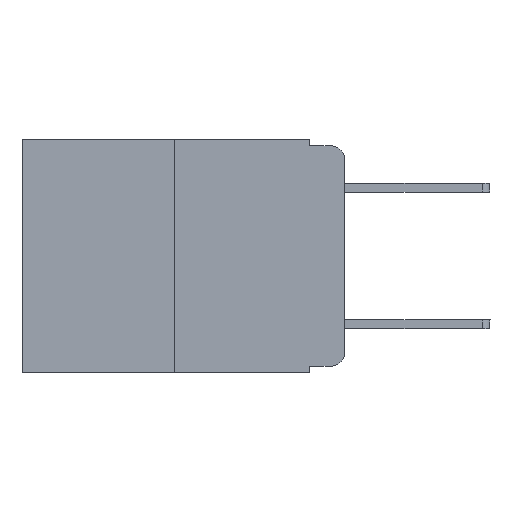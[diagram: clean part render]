
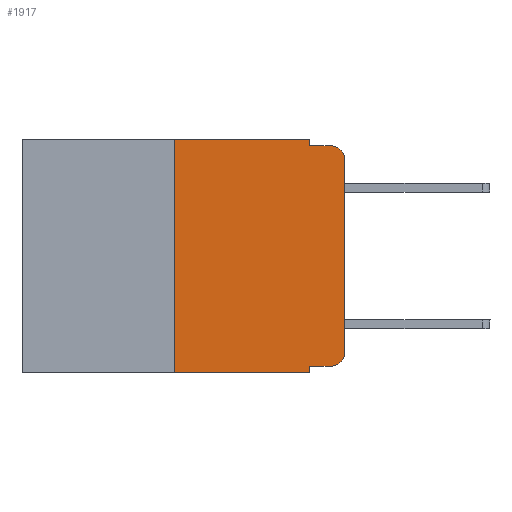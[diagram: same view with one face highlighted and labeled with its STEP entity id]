
A CAD part, left-side view. The second image highlights one B-rep face of the part: STEP entity #1917.
In plain terms, the highlighted planar face has unit normal (-1, 0, 0).
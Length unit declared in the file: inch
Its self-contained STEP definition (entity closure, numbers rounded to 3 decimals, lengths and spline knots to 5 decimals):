
#422 = CARTESIAN_POINT ( 'NONE',  ( 0., 0.02, -0.01 ) ) ;
#666 = ORIENTED_EDGE ( 'NONE', *, *, #4381, .T. ) ;
#1009 = CARTESIAN_POINT ( 'NONE',  ( 0., 0.051, 0. ) ) ;
#1027 = DIRECTION ( 'NONE',  ( 0., -1., 0. ) ) ;
#1063 = CARTESIAN_POINT ( 'NONE',  ( 0., 0.473, 0. ) ) ;
#1115 = ORIENTED_EDGE ( 'NONE', *, *, #6972, .F. ) ;
#1602 = PLANE ( 'NONE',  #3315 ) ;
#1678 = DIRECTION ( 'NONE',  ( 0., -1., 0. ) ) ;
#1718 = EDGE_CURVE ( 'NONE', #6401, #4799, #1751, .T. ) ;
#1751 = LINE ( 'NONE', #2748, #5522 ) ;
#1917 = ADVANCED_FACE ( 'NONE', ( #4671 ), #1602, .F. ) ;
#1966 = DIRECTION ( 'NONE',  ( 0., 0., -1. ) ) ;
#2652 = CARTESIAN_POINT ( 'NONE',  ( 0., 0.051, -0.01 ) ) ;
#2748 = CARTESIAN_POINT ( 'NONE',  ( 0., 0.473, -0.343 ) ) ;
#2893 = CIRCLE ( 'NONE', #5453, 0.02 ) ;
#3029 = VERTEX_POINT ( 'NONE', #7364 ) ;
#3074 = EDGE_CURVE ( 'NONE', #6401, #11103, #7754, .T. ) ;
#3315 = AXIS2_PLACEMENT_3D ( 'NONE', #6069, #7939, #7897 ) ;
#3561 = DIRECTION ( 'NONE',  ( 0., -1., 0. ) ) ;
#3565 = VERTEX_POINT ( 'NONE', #10255 ) ;
#3640 = VECTOR ( 'NONE', #1678, 39.37008 ) ;
#3647 = LINE ( 'NONE', #7190, #3640 ) ;
#3784 = CARTESIAN_POINT ( 'NONE',  ( 0., 0.25, 0. ) ) ;
#4093 = EDGE_CURVE ( 'NONE', #3565, #3029, #3647, .T. ) ;
#4182 = ORIENTED_EDGE ( 'NONE', *, *, #6627, .T. ) ;
#4257 = VERTEX_POINT ( 'NONE', #1009 ) ;
#4373 = DIRECTION ( 'NONE',  ( 0., 0., -1. ) ) ;
#4381 = EDGE_CURVE ( 'NONE', #5866, #6179, #5991, .T. ) ;
#4470 = LINE ( 'NONE', #5321, #10133 ) ;
#4671 = FACE_OUTER_BOUND ( 'NONE', #10088, .T. ) ;
#4758 = ORIENTED_EDGE ( 'NONE', *, *, #3074, .F. ) ;
#4799 = VERTEX_POINT ( 'NONE', #10731 ) ;
#4869 = LINE ( 'NONE', #2652, #9124 ) ;
#5321 = CARTESIAN_POINT ( 'NONE',  ( 0., 0.051, 0. ) ) ;
#5339 = CARTESIAN_POINT ( 'NONE',  ( 0., 0., -0.03 ) ) ;
#5453 = AXIS2_PLACEMENT_3D ( 'NONE', #11638, #9806, #4373 ) ;
#5522 = VECTOR ( 'NONE', #1027, 39.37008 ) ;
#5866 = VERTEX_POINT ( 'NONE', #5339 ) ;
#5936 = ORIENTED_EDGE ( 'NONE', *, *, #1718, .T. ) ;
#5991 = CIRCLE ( 'NONE', #9446, 0.02 ) ;
#6069 = CARTESIAN_POINT ( 'NONE',  ( 0., 0.473, 0. ) ) ;
#6179 = VERTEX_POINT ( 'NONE', #422 ) ;
#6208 = VECTOR ( 'NONE', #7848, 39.37008 ) ;
#6345 = CARTESIAN_POINT ( 'NONE',  ( 0., 0.25, 0. ) ) ;
#6401 = VERTEX_POINT ( 'NONE', #10769 ) ;
#6585 = CARTESIAN_POINT ( 'NONE',  ( 0., 0.02, -0.03 ) ) ;
#6627 = EDGE_CURVE ( 'NONE', #9857, #5866, #6935, .T. ) ;
#6935 = LINE ( 'NONE', #6980, #6208 ) ;
#6972 = EDGE_CURVE ( 'NONE', #4257, #10624, #4470, .T. ) ;
#6980 = CARTESIAN_POINT ( 'NONE',  ( 0., 0., 0. ) ) ;
#7053 = EDGE_CURVE ( 'NONE', #10624, #6179, #4869, .T. ) ;
#7190 = CARTESIAN_POINT ( 'NONE',  ( 0., 0.051, -0.333 ) ) ;
#7230 = DIRECTION ( 'NONE',  ( 0., 0., -1. ) ) ;
#7336 = VECTOR ( 'NONE', #9992, 39.37008 ) ;
#7364 = CARTESIAN_POINT ( 'NONE',  ( 0., 0.02, -0.333 ) ) ;
#7394 = VECTOR ( 'NONE', #9246, 39.37008 ) ;
#7591 = EDGE_CURVE ( 'NONE', #3029, #9857, #2893, .T. ) ;
#7659 = ORIENTED_EDGE ( 'NONE', *, *, #9322, .F. ) ;
#7754 = LINE ( 'NONE', #3784, #7336 ) ;
#7792 = ORIENTED_EDGE ( 'NONE', *, *, #4093, .T. ) ;
#7848 = DIRECTION ( 'NONE',  ( 0., 0., 1. ) ) ;
#7897 = DIRECTION ( 'NONE',  ( 0., 0., -1. ) ) ;
#7906 = ORIENTED_EDGE ( 'NONE', *, *, #7053, .F. ) ;
#7939 = DIRECTION ( 'NONE',  ( 1., 0., 0. ) ) ;
#8043 = EDGE_CURVE ( 'NONE', #3565, #4799, #11002, .T. ) ;
#9120 = VECTOR ( 'NONE', #10081, 39.37008 ) ;
#9124 = VECTOR ( 'NONE', #3561, 39.37008 ) ;
#9246 = DIRECTION ( 'NONE',  ( 0., -1., 0. ) ) ;
#9322 = EDGE_CURVE ( 'NONE', #11103, #4257, #10823, .T. ) ;
#9446 = AXIS2_PLACEMENT_3D ( 'NONE', #6585, #10192, #1966 ) ;
#9806 = DIRECTION ( 'NONE',  ( -1., 0., 0. ) ) ;
#9857 = VERTEX_POINT ( 'NONE', #10928 ) ;
#9975 = ORIENTED_EDGE ( 'NONE', *, *, #8043, .F. ) ;
#9992 = DIRECTION ( 'NONE',  ( 0., 0., 1. ) ) ;
#10081 = DIRECTION ( 'NONE',  ( 0., 0., -1. ) ) ;
#10088 = EDGE_LOOP ( 'NONE', ( #4182, #666, #7906, #1115, #7659, #4758, #5936, #9975, #7792, #10311 ) ) ;
#10133 = VECTOR ( 'NONE', #7230, 39.37008 ) ;
#10192 = DIRECTION ( 'NONE',  ( -1., 0., 0. ) ) ;
#10255 = CARTESIAN_POINT ( 'NONE',  ( 0., 0.051, -0.333 ) ) ;
#10311 = ORIENTED_EDGE ( 'NONE', *, *, #7591, .T. ) ;
#10624 = VERTEX_POINT ( 'NONE', #11199 ) ;
#10731 = CARTESIAN_POINT ( 'NONE',  ( 0., 0.051, -0.343 ) ) ;
#10769 = CARTESIAN_POINT ( 'NONE',  ( 0., 0.25, -0.343 ) ) ;
#10823 = LINE ( 'NONE', #1063, #7394 ) ;
#10928 = CARTESIAN_POINT ( 'NONE',  ( 0., 0., -0.313 ) ) ;
#11002 = LINE ( 'NONE', #11024, #9120 ) ;
#11024 = CARTESIAN_POINT ( 'NONE',  ( 0., 0.051, 0. ) ) ;
#11103 = VERTEX_POINT ( 'NONE', #6345 ) ;
#11199 = CARTESIAN_POINT ( 'NONE',  ( 0., 0.051, -0.01 ) ) ;
#11638 = CARTESIAN_POINT ( 'NONE',  ( 0., 0.02, -0.313 ) ) ;
